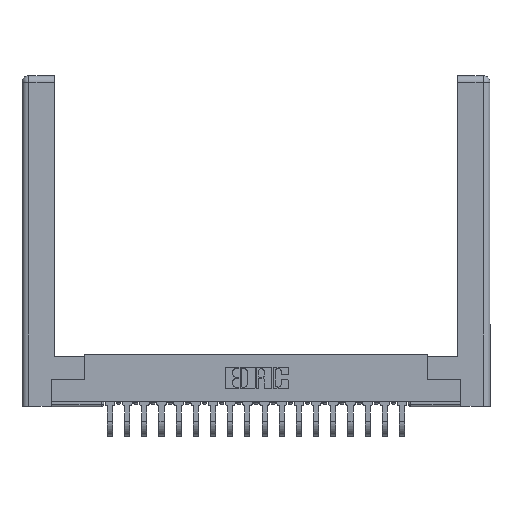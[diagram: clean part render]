
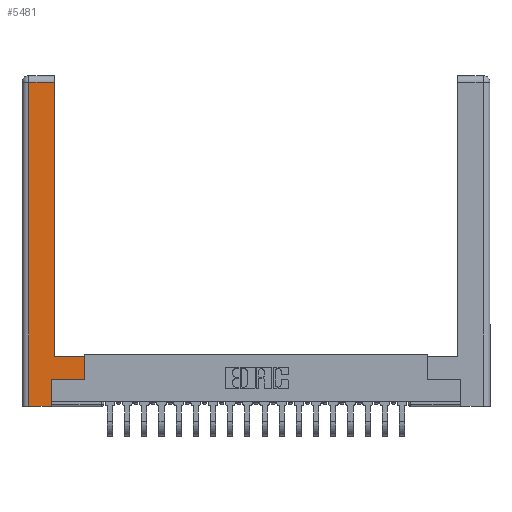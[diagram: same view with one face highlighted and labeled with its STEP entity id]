
A CAD part, top view. The second image highlights one B-rep face of the part: STEP entity #5481.
In plain terms, the highlighted planar face has unit normal (0, 0, 1).
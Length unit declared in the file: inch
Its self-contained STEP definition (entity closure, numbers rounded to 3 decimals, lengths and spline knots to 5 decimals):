
#32 = CARTESIAN_POINT ( 'NONE',  ( 0.0615, 0., 0. ) ) ;
#147 = EDGE_CURVE ( 'NONE', #9154, #16192, #19634, .T. ) ;
#779 = CARTESIAN_POINT ( 'NONE',  ( 0.295, 2.94, 0. ) ) ;
#1141 = EDGE_CURVE ( 'NONE', #12205, #2140, #18172, .T. ) ;
#1347 = VECTOR ( 'NONE', #12492, 39.37008 ) ;
#1571 = VERTEX_POINT ( 'NONE', #10198 ) ;
#1656 = CARTESIAN_POINT ( 'NONE',  ( 0.295, 0.45, 0. ) ) ;
#2063 = DIRECTION ( 'NONE',  ( 0., 0., -1. ) ) ;
#2140 = VERTEX_POINT ( 'NONE', #779 ) ;
#2286 = ORIENTED_EDGE ( 'NONE', *, *, #1141, .T. ) ;
#2427 = LINE ( 'NONE', #10641, #6569 ) ;
#2551 = CARTESIAN_POINT ( 'NONE',  ( 0.0615, 2.94, 0. ) ) ;
#2596 = VECTOR ( 'NONE', #9924, 39.37008 ) ;
#3079 = VECTOR ( 'NONE', #10222, 39.37008 ) ;
#3720 = EDGE_CURVE ( 'NONE', #10823, #1571, #11757, .T. ) ;
#3885 = EDGE_CURVE ( 'NONE', #4970, #10823, #4282, .T. ) ;
#3975 = LINE ( 'NONE', #15829, #15325 ) ;
#4282 = LINE ( 'NONE', #20728, #1347 ) ;
#4773 = ORIENTED_EDGE ( 'NONE', *, *, #3885, .T. ) ;
#4780 = VECTOR ( 'NONE', #12047, 39.37008 ) ;
#4970 = VERTEX_POINT ( 'NONE', #32 ) ;
#5060 = EDGE_CURVE ( 'NONE', #6613, #4970, #2427, .T. ) ;
#5466 = DIRECTION ( 'NONE',  ( -1., 0., 0. ) ) ;
#5481 = ADVANCED_FACE ( 'NONE', ( #13267 ), #8556, .F. ) ;
#5502 = ORIENTED_EDGE ( 'NONE', *, *, #5554, .T. ) ;
#5554 = EDGE_CURVE ( 'NONE', #16192, #12205, #3975, .T. ) ;
#5827 = DIRECTION ( 'NONE',  ( 0., -1., 0. ) ) ;
#6480 = DIRECTION ( 'NONE',  ( 1., 0., 0. ) ) ;
#6569 = VECTOR ( 'NONE', #5827, 39.37008 ) ;
#6613 = VERTEX_POINT ( 'NONE', #8034 ) ;
#7001 = ORIENTED_EDGE ( 'NONE', *, *, #147, .T. ) ;
#7263 = DIRECTION ( 'NONE',  ( -1., 0., 0. ) ) ;
#8034 = CARTESIAN_POINT ( 'NONE',  ( 0.0615, 2.94, 0. ) ) ;
#8089 = ORIENTED_EDGE ( 'NONE', *, *, #20151, .T. ) ;
#8556 = PLANE ( 'NONE',  #13244 ) ;
#9154 = VERTEX_POINT ( 'NONE', #13209 ) ;
#9924 = DIRECTION ( 'NONE',  ( 0., 1., 0. ) ) ;
#10046 = DIRECTION ( 'NONE',  ( 0., 1., 0. ) ) ;
#10198 = CARTESIAN_POINT ( 'NONE',  ( 0.265, 0.245, 0. ) ) ;
#10222 = DIRECTION ( 'NONE',  ( 0., 1., 0. ) ) ;
#10641 = CARTESIAN_POINT ( 'NONE',  ( 0.0615, 0., 0. ) ) ;
#10823 = VERTEX_POINT ( 'NONE', #14828 ) ;
#11757 = LINE ( 'NONE', #18612, #17368 ) ;
#12047 = DIRECTION ( 'NONE',  ( -1., 0., 0. ) ) ;
#12205 = VERTEX_POINT ( 'NONE', #1656 ) ;
#12241 = VECTOR ( 'NONE', #6480, 39.37008 ) ;
#12492 = DIRECTION ( 'NONE',  ( 1., 0., 0. ) ) ;
#12852 = EDGE_LOOP ( 'NONE', ( #2286, #8089, #20081, #4773, #15390, #17647, #7001, #5502 ) ) ;
#13209 = CARTESIAN_POINT ( 'NONE',  ( 0.565, 0.245, 0. ) ) ;
#13244 = AXIS2_PLACEMENT_3D ( 'NONE', #18615, #2063, #5466 ) ;
#13267 = FACE_OUTER_BOUND ( 'NONE', #12852, .T. ) ;
#13342 = LINE ( 'NONE', #19748, #12241 ) ;
#13768 = LINE ( 'NONE', #2551, #4780 ) ;
#14828 = CARTESIAN_POINT ( 'NONE',  ( 0.265, 0., 0. ) ) ;
#15325 = VECTOR ( 'NONE', #7263, 39.37008 ) ;
#15390 = ORIENTED_EDGE ( 'NONE', *, *, #3720, .T. ) ;
#15661 = CARTESIAN_POINT ( 'NONE',  ( 0.565, 0.45, 0. ) ) ;
#15829 = CARTESIAN_POINT ( 'NONE',  ( 0.295, 0.45, 0. ) ) ;
#16192 = VERTEX_POINT ( 'NONE', #15661 ) ;
#16328 = CARTESIAN_POINT ( 'NONE',  ( 0.565, 0.45, 0. ) ) ;
#17368 = VECTOR ( 'NONE', #10046, 39.37008 ) ;
#17647 = ORIENTED_EDGE ( 'NONE', *, *, #18656, .T. ) ;
#18172 = LINE ( 'NONE', #19888, #2596 ) ;
#18612 = CARTESIAN_POINT ( 'NONE',  ( 0.265, 0.245, 0. ) ) ;
#18615 = CARTESIAN_POINT ( 'NONE',  ( 0., 0., 0. ) ) ;
#18656 = EDGE_CURVE ( 'NONE', #1571, #9154, #13342, .T. ) ;
#19634 = LINE ( 'NONE', #16328, #3079 ) ;
#19748 = CARTESIAN_POINT ( 'NONE',  ( 0.565, 0.245, 0. ) ) ;
#19888 = CARTESIAN_POINT ( 'NONE',  ( 0.295, 3., 0. ) ) ;
#20081 = ORIENTED_EDGE ( 'NONE', *, *, #5060, .T. ) ;
#20151 = EDGE_CURVE ( 'NONE', #2140, #6613, #13768, .T. ) ;
#20728 = CARTESIAN_POINT ( 'NONE',  ( 0.265, 0., 0. ) ) ;
